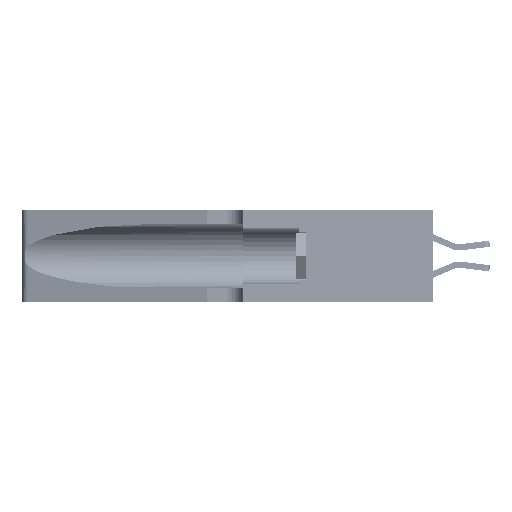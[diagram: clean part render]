
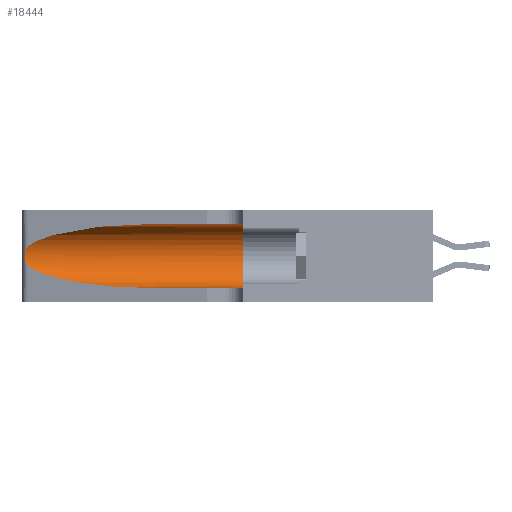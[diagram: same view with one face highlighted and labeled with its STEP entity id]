
A CAD part, left-side view. The second image highlights one B-rep face of the part: STEP entity #18444.
In plain terms, the highlighted cylindrical face has radius 3.308 mm (diameter 6.617 mm), a partial arc.
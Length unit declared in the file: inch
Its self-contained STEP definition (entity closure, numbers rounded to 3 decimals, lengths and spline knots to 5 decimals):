
#632 = DIRECTION ( 'NONE',  ( 0., 0., -1. ) ) ;
#1117 = CARTESIAN_POINT ( 'NONE',  ( 0.25487, 1.22718, 0.22369 ) ) ;
#1544 = CARTESIAN_POINT ( 'NONE',  ( 0.25639, 1.23184, 0.21858 ) ) ;
#1866 = CARTESIAN_POINT ( 'NONE',  ( 0.1305, 1.61858, 0.31525 ) ) ;
#2113 = B_SPLINE_CURVE_WITH_KNOTS ( 'NONE', 3,
 ( #13646, #36399, #1544, #2226, #16254, #41934, #3593, #26340, #32399, #34622, #41329, #11534, #16656, #29163 ),
 .UNSPECIFIED., .F., .F.,
 ( 4, 2, 2, 2, 2, 2, 4 ),
 ( 0., 0.00027, 0.00053, 0.00107, 0.0016, 0.00187, 0.00214 ),
 .UNSPECIFIED. ) ;
#2226 = CARTESIAN_POINT ( 'NONE',  ( 0.25787, 1.23484, 0.2124 ) ) ;
#3243 = DIRECTION ( 'NONE',  ( 0., 0., 1. ) ) ;
#3593 = CARTESIAN_POINT ( 'NONE',  ( 0.26075, 1.23896, 0.19203 ) ) ;
#6632 = DIRECTION ( 'NONE',  ( 0., -1., 0. ) ) ;
#6634 = CARTESIAN_POINT ( 'NONE',  ( 0.25487, 1.22718, 0.14631 ) ) ;
#7334 = AXIS2_PLACEMENT_3D ( 'NONE', #38382, #22713, #3243 ) ;
#7365 = CARTESIAN_POINT ( 'NONE',  ( 0.18966, 0.96281, 0.31525 ) ) ;
#7405 = CYLINDRICAL_SURFACE ( 'NONE', #31081, 0.13025 ) ;
#7865 = VERTEX_POINT ( 'NONE', #33679 ) ;
#8642 = CARTESIAN_POINT ( 'NONE',  ( 0.1305, 1.61858, 0.05475 ) ) ;
#9742 = VERTEX_POINT ( 'NONE', #1117 ) ;
#9766 = VERTEX_POINT ( 'NONE', #13565 ) ;
#10439 = VERTEX_POINT ( 'NONE', #6634 ) ;
#10657 = CARTESIAN_POINT ( 'NONE',  ( 0.2373, 1.15595, 0.28018 ) ) ;
#10808 = CARTESIAN_POINT ( 'NONE',  ( 0.1305, 0.72297, 0.31525 ) ) ;
#11534 = CARTESIAN_POINT ( 'NONE',  ( 0.25639, 1.23186, 0.15144 ) ) ;
#11629 = DIRECTION ( 'NONE',  ( 0., -1., 0. ) ) ;
#11794 = ORIENTED_EDGE ( 'NONE', *, *, #39026, .T. ) ;
#12290 = EDGE_CURVE ( 'NONE', #9742, #10439, #2113, .T. ) ;
#12741 = CARTESIAN_POINT ( 'NONE',  ( 0.1305, 0.72297, 0.05475 ) ) ;
#13565 = CARTESIAN_POINT ( 'NONE',  ( 0.1305, 0.35, 0.31525 ) ) ;
#13646 = CARTESIAN_POINT ( 'NONE',  ( 0.25487, 1.22718, 0.22369 ) ) ;
#16052 = CARTESIAN_POINT ( 'NONE',  ( 0.25487, 1.22718, 0.14631 ) ) ;
#16254 = CARTESIAN_POINT ( 'NONE',  ( 0.25854, 1.2359, 0.20912 ) ) ;
#16656 = CARTESIAN_POINT ( 'NONE',  ( 0.25555, 1.22993, 0.14849 ) ) ;
#16768 = ORIENTED_EDGE ( 'NONE', *, *, #40352, .T. ) ;
#17000 = ORIENTED_EDGE ( 'NONE', *, *, #38416, .T. ) ;
#18444 = ADVANCED_FACE ( 'NONE', ( #19204 ), #7405, .F. ) ;
#19204 = FACE_OUTER_BOUND ( 'NONE', #20669, .T. ) ;
#19231 = ORIENTED_EDGE ( 'NONE', *, *, #23755, .F. ) ;
#20669 = EDGE_LOOP ( 'NONE', ( #16768, #23889, #11794, #17000, #26396, #19231 ) ) ;
#22692 = LINE ( 'NONE', #8642, #23693 ) ;
#22713 = DIRECTION ( 'NONE',  ( 0., 1., 0. ) ) ;
#23287 = CARTESIAN_POINT ( 'NONE',  ( 0.1305, 1.61858, 0.185 ) ) ;
#23693 = VECTOR ( 'NONE', #31432, 39.37008 ) ;
#23755 = EDGE_CURVE ( 'NONE', #25983, #9766, #29076, .T. ) ;
#23889 = ORIENTED_EDGE ( 'NONE', *, *, #12290, .T. ) ;
#25025 = CARTESIAN_POINT ( 'NONE',  ( 0.2373, 1.15595, 0.08982 ) ) ;
#25983 = VERTEX_POINT ( 'NONE', #10808 ) ;
#26340 = CARTESIAN_POINT ( 'NONE',  ( 0.26075, 1.23896, 0.178 ) ) ;
#26396 = ORIENTED_EDGE ( 'NONE', *, *, #31797, .F. ) ;
#26566 =( BOUNDED_CURVE ( )  B_SPLINE_CURVE ( 3, ( #40150, #7365, #10657, #33303 ),
 .UNSPECIFIED., .F., .T. ) 
 B_SPLINE_CURVE_WITH_KNOTS ( ( 4, 4 ),
 ( 1.5708, 2.84003 ),
 .UNSPECIFIED. ) 
 CURVE ( )  GEOMETRIC_REPRESENTATION_ITEM ( )  RATIONAL_B_SPLINE_CURVE ( ( 1., 0.87, 0.87, 1. ) ) 
 REPRESENTATION_ITEM ( '' )  );
#29076 = LINE ( 'NONE', #1866, #35715 ) ;
#29163 = CARTESIAN_POINT ( 'NONE',  ( 0.25487, 1.22718, 0.14631 ) ) ;
#29681 =( BOUNDED_CURVE ( )  B_SPLINE_CURVE ( 3, ( #16052, #25025, #34677, #12741 ),
 .UNSPECIFIED., .F., .T. ) 
 B_SPLINE_CURVE_WITH_KNOTS ( ( 4, 4 ),
 ( 3.44316, 4.71239 ),
 .UNSPECIFIED. ) 
 CURVE ( )  GEOMETRIC_REPRESENTATION_ITEM ( )  RATIONAL_B_SPLINE_CURVE ( ( 1., 0.87, 0.87, 1. ) ) 
 REPRESENTATION_ITEM ( '' )  );
#31081 = AXIS2_PLACEMENT_3D ( 'NONE', #23287, #6632, #632 ) ;
#31432 = DIRECTION ( 'NONE',  ( 0., -1., 0. ) ) ;
#31797 = EDGE_CURVE ( 'NONE', #9766, #40034, #33438, .T. ) ;
#32399 = CARTESIAN_POINT ( 'NONE',  ( 0.26017, 1.23833, 0.17102 ) ) ;
#33303 = CARTESIAN_POINT ( 'NONE',  ( 0.25487, 1.22718, 0.22369 ) ) ;
#33438 = CIRCLE ( 'NONE', #7334, 0.13025 ) ;
#33679 = CARTESIAN_POINT ( 'NONE',  ( 0.1305, 0.72297, 0.05475 ) ) ;
#34622 = CARTESIAN_POINT ( 'NONE',  ( 0.25856, 1.23593, 0.16098 ) ) ;
#34677 = CARTESIAN_POINT ( 'NONE',  ( 0.18966, 0.96281, 0.05475 ) ) ;
#35715 = VECTOR ( 'NONE', #11629, 39.37008 ) ;
#36399 = CARTESIAN_POINT ( 'NONE',  ( 0.25555, 1.22994, 0.2215 ) ) ;
#38382 = CARTESIAN_POINT ( 'NONE',  ( 0.1305, 0.35, 0.185 ) ) ;
#38416 = EDGE_CURVE ( 'NONE', #7865, #40034, #22692, .T. ) ;
#38771 = CARTESIAN_POINT ( 'NONE',  ( 0.1305, 0.35, 0.05475 ) ) ;
#39026 = EDGE_CURVE ( 'NONE', #10439, #7865, #29681, .T. ) ;
#40034 = VERTEX_POINT ( 'NONE', #38771 ) ;
#40150 = CARTESIAN_POINT ( 'NONE',  ( 0.1305, 0.72297, 0.31525 ) ) ;
#40352 = EDGE_CURVE ( 'NONE', #25983, #9742, #26566, .T. ) ;
#41329 = CARTESIAN_POINT ( 'NONE',  ( 0.25789, 1.23486, 0.15765 ) ) ;
#41934 = CARTESIAN_POINT ( 'NONE',  ( 0.26018, 1.23835, 0.19895 ) ) ;
